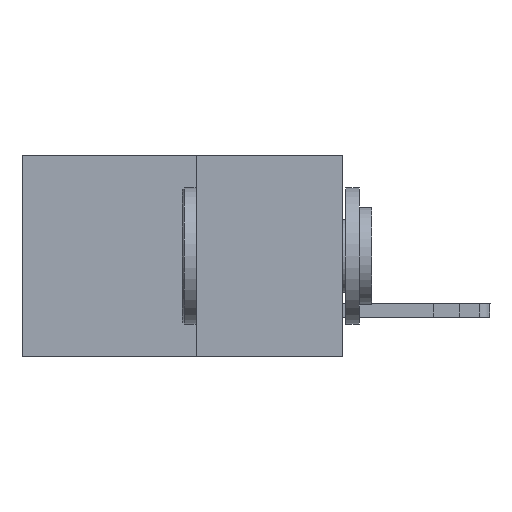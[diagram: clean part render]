
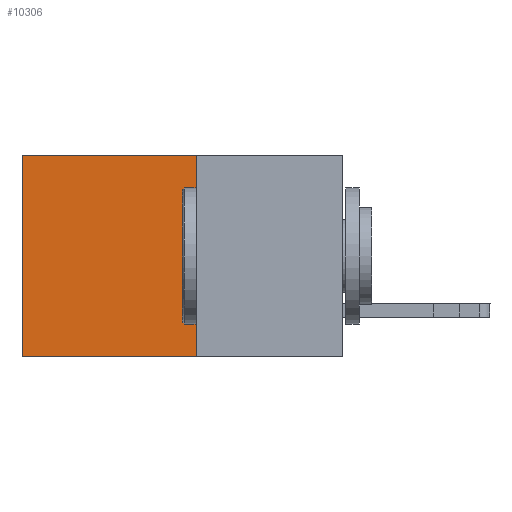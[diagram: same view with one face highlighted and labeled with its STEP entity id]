
A CAD part, left-side view. The second image highlights one B-rep face of the part: STEP entity #10306.
In plain terms, the highlighted planar face has unit normal (-1, 0, 0).
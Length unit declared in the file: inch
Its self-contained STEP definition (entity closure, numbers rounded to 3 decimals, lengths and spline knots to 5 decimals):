
#13 = CARTESIAN_POINT ( 'NONE',  ( 0.277, 0.27, 0. ) ) ;
#287 = CARTESIAN_POINT ( 'NONE',  ( 0.277, 0.59, 0. ) ) ;
#466 = VECTOR ( 'NONE', #4488, 39.37008 ) ;
#835 = VERTEX_POINT ( 'NONE', #12645 ) ;
#3291 = EDGE_CURVE ( 'NONE', #8507, #8661, #4585, .T. ) ;
#3527 = VECTOR ( 'NONE', #8378, 39.37008 ) ;
#3835 = DIRECTION ( 'NONE',  ( 0., 1., 0. ) ) ;
#3906 = CARTESIAN_POINT ( 'NONE',  ( 0.277, 0.27, 0. ) ) ;
#3948 = EDGE_CURVE ( 'NONE', #8661, #835, #7159, .T. ) ;
#4312 = PLANE ( 'NONE',  #14223 ) ;
#4488 = DIRECTION ( 'NONE',  ( 0., 0., -1. ) ) ;
#4585 = LINE ( 'NONE', #3906, #7718 ) ;
#4608 = ORIENTED_EDGE ( 'NONE', *, *, #3948, .T. ) ;
#4736 = VECTOR ( 'NONE', #9423, 39.37008 ) ;
#5754 = VERTEX_POINT ( 'NONE', #7613 ) ;
#6467 = ORIENTED_EDGE ( 'NONE', *, *, #11271, .F. ) ;
#6651 = LINE ( 'NONE', #9495, #3527 ) ;
#6696 = DIRECTION ( 'NONE',  ( 0., 0., -1. ) ) ;
#7051 = FACE_OUTER_BOUND ( 'NONE', #7137, .T. ) ;
#7137 = EDGE_LOOP ( 'NONE', ( #4608, #6467, #9541, #13028 ) ) ;
#7159 = LINE ( 'NONE', #14123, #4736 ) ;
#7613 = CARTESIAN_POINT ( 'NONE',  ( 0.277, 0.27, -0.37 ) ) ;
#7718 = VECTOR ( 'NONE', #3835, 39.37008 ) ;
#7825 = CARTESIAN_POINT ( 'NONE',  ( 0.277, 0.27, -0.37 ) ) ;
#8378 = DIRECTION ( 'NONE',  ( 0., 1., 0. ) ) ;
#8507 = VERTEX_POINT ( 'NONE', #13 ) ;
#8661 = VERTEX_POINT ( 'NONE', #287 ) ;
#9423 = DIRECTION ( 'NONE',  ( 0., 0., -1. ) ) ;
#9495 = CARTESIAN_POINT ( 'NONE',  ( 0.277, 0.27, -0.37 ) ) ;
#9541 = ORIENTED_EDGE ( 'NONE', *, *, #14632, .F. ) ;
#10297 = CARTESIAN_POINT ( 'NONE',  ( 0.277, 0.27, -0.37 ) ) ;
#10306 = ADVANCED_FACE ( 'NONE', ( #7051 ), #4312, .F. ) ;
#11271 = EDGE_CURVE ( 'NONE', #5754, #835, #6651, .T. ) ;
#12478 = LINE ( 'NONE', #10297, #466 ) ;
#12645 = CARTESIAN_POINT ( 'NONE',  ( 0.277, 0.59, -0.37 ) ) ;
#13028 = ORIENTED_EDGE ( 'NONE', *, *, #3291, .T. ) ;
#13673 = DIRECTION ( 'NONE',  ( 1., 0., 0. ) ) ;
#14123 = CARTESIAN_POINT ( 'NONE',  ( 0.277, 0.59, -0.37 ) ) ;
#14223 = AXIS2_PLACEMENT_3D ( 'NONE', #7825, #13673, #6696 ) ;
#14632 = EDGE_CURVE ( 'NONE', #8507, #5754, #12478, .T. ) ;
